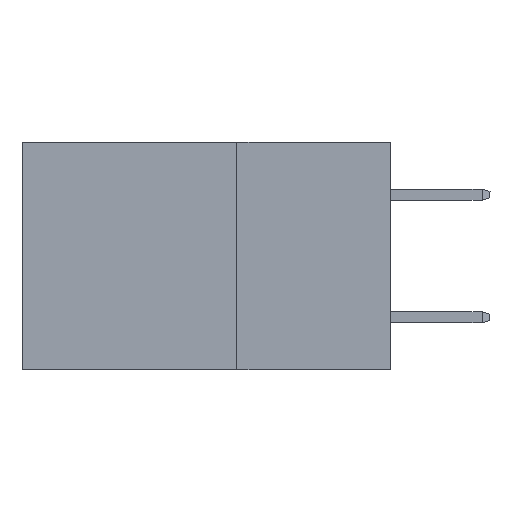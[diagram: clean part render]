
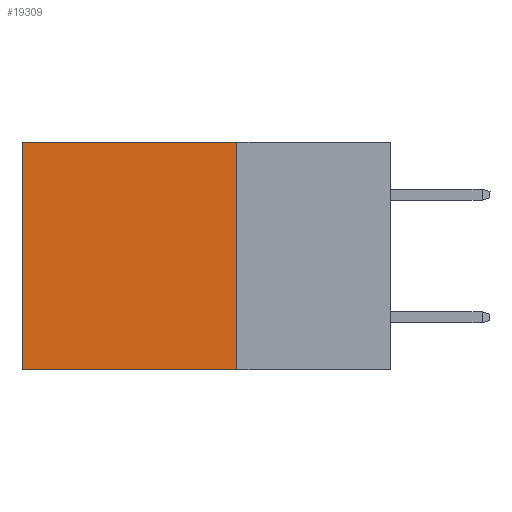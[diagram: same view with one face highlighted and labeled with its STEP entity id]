
A CAD part, left-side view. The second image highlights one B-rep face of the part: STEP entity #19309.
In plain terms, the highlighted planar face has unit normal (-1, 0, 0).
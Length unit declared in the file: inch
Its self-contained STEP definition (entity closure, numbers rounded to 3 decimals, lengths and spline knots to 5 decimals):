
#143 = LINE ( 'NONE', #20456, #21018 ) ;
#414 = AXIS2_PLACEMENT_3D ( 'NONE', #12220, #20347, #10629 ) ;
#1327 = DIRECTION ( 'NONE',  ( 0., 1., 0. ) ) ;
#1672 = ORIENTED_EDGE ( 'NONE', *, *, #4128, .F. ) ;
#1758 = EDGE_CURVE ( 'NONE', #7294, #16251, #2057, .T. ) ;
#2057 = LINE ( 'NONE', #9678, #19090 ) ;
#2514 = DIRECTION ( 'NONE',  ( 0., 0., -1. ) ) ;
#3338 = LINE ( 'NONE', #10924, #15467 ) ;
#3523 = EDGE_CURVE ( 'NONE', #16251, #11210, #3338, .T. ) ;
#3958 = VECTOR ( 'NONE', #19893, 39.37008 ) ;
#4128 = EDGE_CURVE ( 'NONE', #7294, #5920, #143, .T. ) ;
#5920 = VERTEX_POINT ( 'NONE', #16000 ) ;
#7294 = VERTEX_POINT ( 'NONE', #14670 ) ;
#8481 = CARTESIAN_POINT ( 'NONE',  ( 0.2875, 0.25, -0.37 ) ) ;
#8963 = PLANE ( 'NONE',  #414 ) ;
#9071 = DIRECTION ( 'NONE',  ( 0., 0., -1. ) ) ;
#9110 = EDGE_LOOP ( 'NONE', ( #19339, #20166, #1672, #9766 ) ) ;
#9123 = EDGE_CURVE ( 'NONE', #5920, #11210, #12799, .T. ) ;
#9678 = CARTESIAN_POINT ( 'NONE',  ( 0.2875, 0.25, 0. ) ) ;
#9766 = ORIENTED_EDGE ( 'NONE', *, *, #1758, .T. ) ;
#10629 = DIRECTION ( 'NONE',  ( 0., 0., -1. ) ) ;
#10924 = CARTESIAN_POINT ( 'NONE',  ( 0.2875, 0.6, 0. ) ) ;
#11210 = VERTEX_POINT ( 'NONE', #12867 ) ;
#12220 = CARTESIAN_POINT ( 'NONE',  ( 0.2875, 0.25, 0. ) ) ;
#12799 = LINE ( 'NONE', #8481, #3958 ) ;
#12867 = CARTESIAN_POINT ( 'NONE',  ( 0.2875, 0.6, -0.37 ) ) ;
#14670 = CARTESIAN_POINT ( 'NONE',  ( 0.2875, 0.25, 0. ) ) ;
#15467 = VECTOR ( 'NONE', #2514, 39.37008 ) ;
#15700 = CARTESIAN_POINT ( 'NONE',  ( 0.2875, 0.6, 0. ) ) ;
#16000 = CARTESIAN_POINT ( 'NONE',  ( 0.2875, 0.25, -0.37 ) ) ;
#16251 = VERTEX_POINT ( 'NONE', #15700 ) ;
#16637 = FACE_OUTER_BOUND ( 'NONE', #9110, .T. ) ;
#19090 = VECTOR ( 'NONE', #1327, 39.37008 ) ;
#19309 = ADVANCED_FACE ( 'NONE', ( #16637 ), #8963, .F. ) ;
#19339 = ORIENTED_EDGE ( 'NONE', *, *, #3523, .T. ) ;
#19893 = DIRECTION ( 'NONE',  ( 0., 1., 0. ) ) ;
#20166 = ORIENTED_EDGE ( 'NONE', *, *, #9123, .F. ) ;
#20347 = DIRECTION ( 'NONE',  ( 1., 0., 0. ) ) ;
#20456 = CARTESIAN_POINT ( 'NONE',  ( 0.2875, 0.25, 0. ) ) ;
#21018 = VECTOR ( 'NONE', #9071, 39.37008 ) ;
